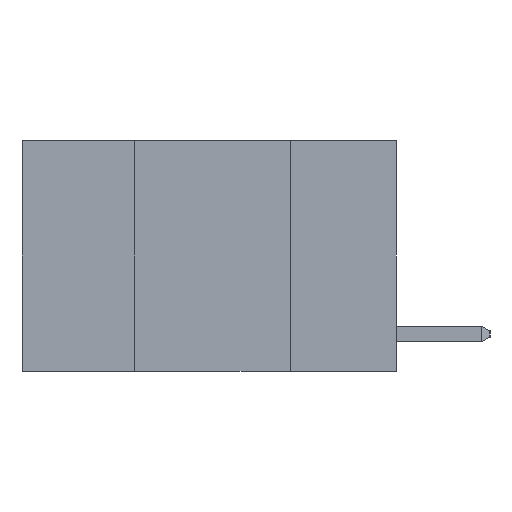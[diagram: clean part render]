
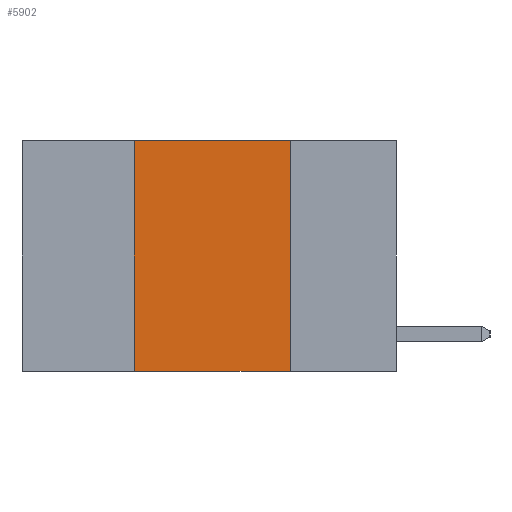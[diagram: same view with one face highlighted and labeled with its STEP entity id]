
A CAD part, left-side view. The second image highlights one B-rep face of the part: STEP entity #5902.
In plain terms, the highlighted planar face has unit normal (-1, 0, 0).
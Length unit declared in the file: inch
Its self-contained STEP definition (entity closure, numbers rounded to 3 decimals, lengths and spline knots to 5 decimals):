
#294 = CARTESIAN_POINT ( 'NONE',  ( 0., 0.17, 0. ) ) ;
#404 = VERTEX_POINT ( 'NONE', #2427 ) ;
#649 = DIRECTION ( 'NONE',  ( 0., 0., 1. ) ) ;
#2001 = VERTEX_POINT ( 'NONE', #11379 ) ;
#2427 = CARTESIAN_POINT ( 'NONE',  ( 0., 0.17, -0.37 ) ) ;
#3162 = VECTOR ( 'NONE', #14228, 39.37008 ) ;
#3742 = CARTESIAN_POINT ( 'NONE',  ( 0., 0.42, 0. ) ) ;
#5902 = ADVANCED_FACE ( 'NONE', ( #14843 ), #13520, .F. ) ;
#5953 = LINE ( 'NONE', #13069, #12352 ) ;
#6365 = CARTESIAN_POINT ( 'NONE',  ( 0., 0.6, 0. ) ) ;
#6460 = ORIENTED_EDGE ( 'NONE', *, *, #9192, .F. ) ;
#7115 = VERTEX_POINT ( 'NONE', #3742 ) ;
#7566 = DIRECTION ( 'NONE',  ( 0., 0., -1. ) ) ;
#7684 = EDGE_CURVE ( 'NONE', #10529, #404, #11992, .T. ) ;
#7905 = EDGE_CURVE ( 'NONE', #2001, #404, #8621, .T. ) ;
#8621 = LINE ( 'NONE', #294, #14589 ) ;
#8965 = CARTESIAN_POINT ( 'NONE',  ( 0., 0.42, -0.37 ) ) ;
#9046 = CARTESIAN_POINT ( 'NONE',  ( 0., 0.42, 0. ) ) ;
#9192 = EDGE_CURVE ( 'NONE', #7115, #2001, #5953, .T. ) ;
#10114 = EDGE_LOOP ( 'NONE', ( #15255, #6460, #10784, #11537 ) ) ;
#10529 = VERTEX_POINT ( 'NONE', #8965 ) ;
#10784 = ORIENTED_EDGE ( 'NONE', *, *, #14191, .F. ) ;
#11379 = CARTESIAN_POINT ( 'NONE',  ( 0., 0.17, 0. ) ) ;
#11537 = ORIENTED_EDGE ( 'NONE', *, *, #7684, .T. ) ;
#11992 = LINE ( 'NONE', #13035, #3162 ) ;
#12352 = VECTOR ( 'NONE', #14255, 39.37008 ) ;
#12926 = AXIS2_PLACEMENT_3D ( 'NONE', #6365, #14735, #7566 ) ;
#13035 = CARTESIAN_POINT ( 'NONE',  ( 0., 0.6, -0.37 ) ) ;
#13069 = CARTESIAN_POINT ( 'NONE',  ( 0., 0.6, 0. ) ) ;
#13493 = DIRECTION ( 'NONE',  ( 0., 0., -1. ) ) ;
#13520 = PLANE ( 'NONE',  #12926 ) ;
#14191 = EDGE_CURVE ( 'NONE', #10529, #7115, #15311, .T. ) ;
#14228 = DIRECTION ( 'NONE',  ( 0., -1., 0. ) ) ;
#14255 = DIRECTION ( 'NONE',  ( 0., -1., 0. ) ) ;
#14589 = VECTOR ( 'NONE', #13493, 39.37008 ) ;
#14735 = DIRECTION ( 'NONE',  ( 1., 0., 0. ) ) ;
#14843 = FACE_OUTER_BOUND ( 'NONE', #10114, .T. ) ;
#14938 = VECTOR ( 'NONE', #649, 39.37008 ) ;
#15255 = ORIENTED_EDGE ( 'NONE', *, *, #7905, .F. ) ;
#15311 = LINE ( 'NONE', #9046, #14938 ) ;
